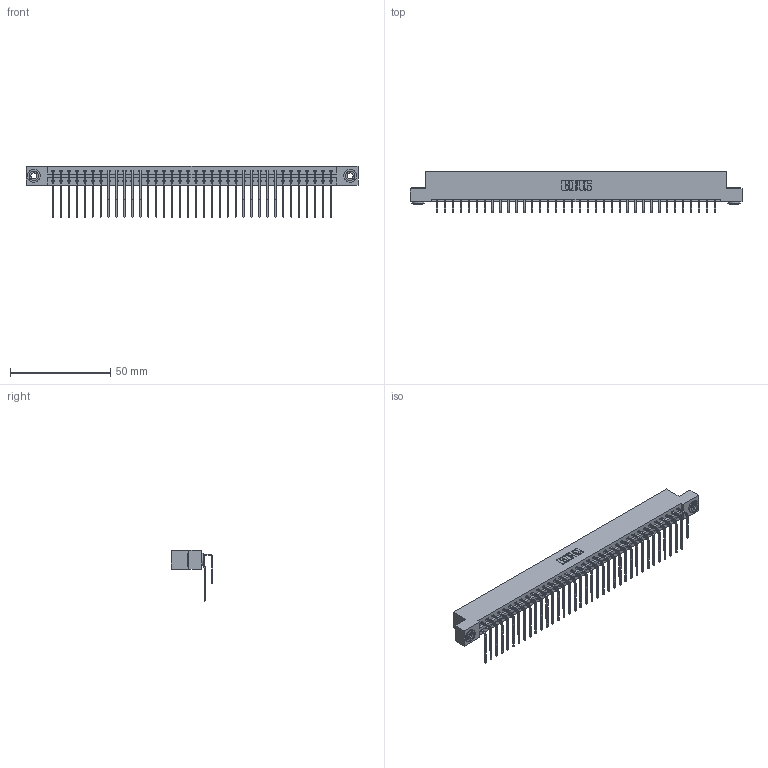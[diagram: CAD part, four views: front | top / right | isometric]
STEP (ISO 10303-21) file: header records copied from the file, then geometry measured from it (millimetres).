
FILE_DESCRIPTION (( 'STEP AP203' ), '1' );
FILE_NAME ('337-072-559-203.STEP', '2019-10-10T03:05:46', ( '' ), ( '' ), 'SwSTEP 2.0', 'SolidWorks 2016', '' );
FILE_SCHEMA (( 'CONFIG_CONTROL_DESIGN' ));
Length unit declared in the file: inch
Products named in the file (5): 345-292-001_558 559 Tail - 1; 345-292-001_559 Tail - 2; 337 Part_Flush Mounting Lugs - 0.156 Dia-TH; 345-250-002_345-250-002-102; 337-072-559-203
Assembly tree (75 placements, depth 2):
  337-072-559-203
    337 Part_Flush Mounting Lugs - 0.156 Dia-TH
    345-292-001_558 559 Tail - 1  x36
    345-292-001_559 Tail - 2  x36
    345-250-002_345-250-002-102  x2
Bounding box: 165.66 x 20.9 x 25.53 mm (x, y, z)
Volume: 17813.3 mm3; surface area: 22389.7 mm2
Topology: 75 solids, 75 shells, 4184 faces, 12411 edges, 8174 vertices
Faces by surface type: plane 2960, cylinder 1216, cone 8
Entity records: 31122 total; most frequent: CARTESIAN_POINT 5268, ORIENTED_EDGE 5146, DIRECTION 4507, EDGE_CURVE 2573, LINE 2381, VECTOR 2381, VERTEX_POINT 1710, AXIS2_PLACEMENT_3D 1063
